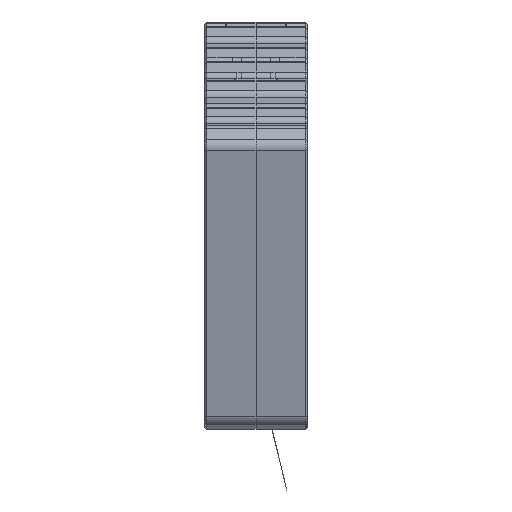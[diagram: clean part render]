
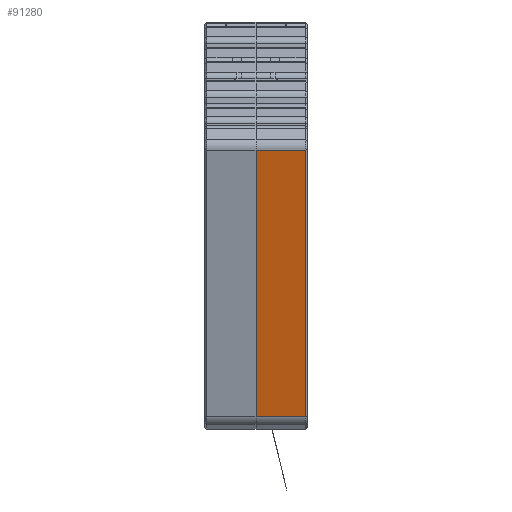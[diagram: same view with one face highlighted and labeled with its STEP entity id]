
A CAD part, front view. The second image highlights one B-rep face of the part: STEP entity #91280.
In plain terms, the highlighted planar face has unit normal (0, -0.97, -0.241).
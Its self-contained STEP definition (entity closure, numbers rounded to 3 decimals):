
#10251 = ORIENTED_EDGE ( 'NONE', *, *, #51086, .F. ) ;
#13747 = ORIENTED_EDGE ( 'NONE', *, *, #161648, .F. ) ;
#14285 = CARTESIAN_POINT ( 'NONE',  ( 0., -144.69, -54.333 ) ) ;
#20130 = AXIS2_PLACEMENT_3D ( 'NONE', #43420, #72739, #122820 ) ;
#20179 = ORIENTED_EDGE ( 'NONE', *, *, #53492, .T. ) ;
#23920 = CARTESIAN_POINT ( 'NONE',  ( 12.252, -144.332, -55.775 ) ) ;
#26085 = DIRECTION ( 'NONE',  ( 0., 0.241, -0.97 ) ) ;
#27195 = LINE ( 'NONE', #37902, #117311 ) ;
#27791 = CARTESIAN_POINT ( 'NONE',  ( 12.252, -160.79, 10.379 ) ) ;
#28555 = VERTEX_POINT ( 'NONE', #86342 ) ;
#36774 = LINE ( 'NONE', #38402, #94343 ) ;
#37902 = CARTESIAN_POINT ( 'NONE',  ( 110.954, -144.332, -55.775 ) ) ;
#38402 = CARTESIAN_POINT ( 'NONE',  ( 12.252, -144.69, -54.333 ) ) ;
#43420 = CARTESIAN_POINT ( 'NONE',  ( 110.954, -144.69, -54.333 ) ) ;
#44082 = CARTESIAN_POINT ( 'NONE',  ( 0., -160.79, 10.379 ) ) ;
#51086 = EDGE_CURVE ( 'NONE', #88022, #86465, #36774, .T. ) ;
#53492 = EDGE_CURVE ( 'NONE', #87107, #28555, #87390, .T. ) ;
#53791 = LINE ( 'NONE', #156395, #106723 ) ;
#67796 = EDGE_LOOP ( 'NONE', ( #13747, #20179, #104746, #10251 ) ) ;
#72739 = DIRECTION ( 'NONE',  ( 0., -0.97, -0.241 ) ) ;
#86342 = CARTESIAN_POINT ( 'NONE',  ( 0., -144.332, -55.775 ) ) ;
#86465 = VERTEX_POINT ( 'NONE', #23920 ) ;
#87107 = VERTEX_POINT ( 'NONE', #44082 ) ;
#87390 = LINE ( 'NONE', #14285, #113268 ) ;
#88022 = VERTEX_POINT ( 'NONE', #27791 ) ;
#91280 = ADVANCED_FACE ( 'NONE', ( #130468 ), #135163, .T. ) ;
#92318 = EDGE_CURVE ( 'NONE', #86465, #28555, #27195, .T. ) ;
#94343 = VECTOR ( 'NONE', #26085, 1000. ) ;
#103882 = DIRECTION ( 'NONE',  ( 1., 0., 0. ) ) ;
#104746 = ORIENTED_EDGE ( 'NONE', *, *, #92318, .F. ) ;
#106723 = VECTOR ( 'NONE', #103882, 1000. ) ;
#113268 = VECTOR ( 'NONE', #139089, 1000. ) ;
#117311 = VECTOR ( 'NONE', #125770, 1000. ) ;
#122820 = DIRECTION ( 'NONE',  ( 0., 0.241, -0.97 ) ) ;
#125770 = DIRECTION ( 'NONE',  ( -1., 0., 0. ) ) ;
#130468 = FACE_OUTER_BOUND ( 'NONE', #67796, .T. ) ;
#135163 = PLANE ( 'NONE',  #20130 ) ;
#139089 = DIRECTION ( 'NONE',  ( 0., 0.241, -0.97 ) ) ;
#156395 = CARTESIAN_POINT ( 'NONE',  ( 110.954, -160.79, 10.379 ) ) ;
#161648 = EDGE_CURVE ( 'NONE', #87107, #88022, #53791, .T. ) ;
